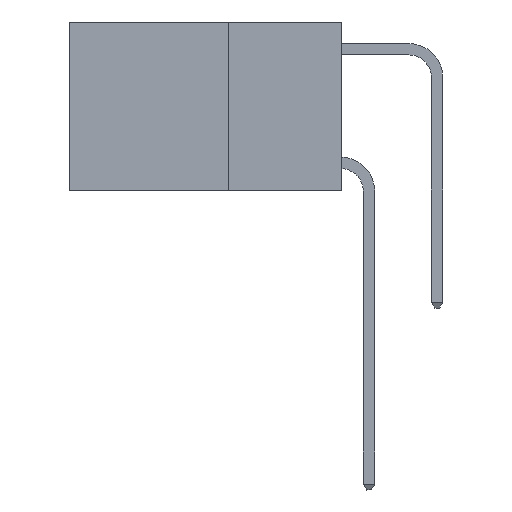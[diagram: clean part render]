
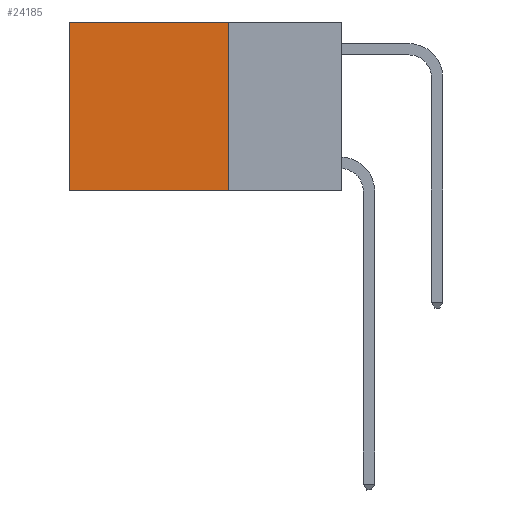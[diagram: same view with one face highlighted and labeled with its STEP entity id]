
A CAD part, left-side view. The second image highlights one B-rep face of the part: STEP entity #24185.
In plain terms, the highlighted planar face has unit normal (-1, 0, 0).
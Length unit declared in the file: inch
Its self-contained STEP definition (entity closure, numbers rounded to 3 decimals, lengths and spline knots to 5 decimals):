
#81 = CARTESIAN_POINT ( 'NONE',  ( 0.2625, 0.6, -0.37 ) ) ;
#1152 = ORIENTED_EDGE ( 'NONE', *, *, #24016, .T. ) ;
#2086 = VECTOR ( 'NONE', #6227, 39.37008 ) ;
#2384 = VERTEX_POINT ( 'NONE', #5807 ) ;
#2871 = CARTESIAN_POINT ( 'NONE',  ( 0.2625, 0.25, 0. ) ) ;
#3083 = EDGE_LOOP ( 'NONE', ( #29100, #20463, #23077, #1152 ) ) ;
#3670 = VECTOR ( 'NONE', #8226, 39.37008 ) ;
#3983 = LINE ( 'NONE', #14456, #13531 ) ;
#4513 = VERTEX_POINT ( 'NONE', #81 ) ;
#5807 = CARTESIAN_POINT ( 'NONE',  ( 0.2625, 0.25, 0. ) ) ;
#6227 = DIRECTION ( 'NONE',  ( 0., 1., 0. ) ) ;
#7816 = LINE ( 'NONE', #2871, #2086 ) ;
#7934 = LINE ( 'NONE', #18418, #25900 ) ;
#8226 = DIRECTION ( 'NONE',  ( 0., 1., 0. ) ) ;
#9347 = EDGE_CURVE ( 'NONE', #2384, #14839, #3983, .T. ) ;
#10185 = VERTEX_POINT ( 'NONE', #24954 ) ;
#10388 = CARTESIAN_POINT ( 'NONE',  ( 0.2625, 0.25, -0.37 ) ) ;
#10631 = CARTESIAN_POINT ( 'NONE',  ( 0.2625, 0.25, -0.37 ) ) ;
#11155 = LINE ( 'NONE', #10631, #3670 ) ;
#11857 = DIRECTION ( 'NONE',  ( 0., 0., -1. ) ) ;
#13272 = DIRECTION ( 'NONE',  ( 0., 0., -1. ) ) ;
#13531 = VECTOR ( 'NONE', #11857, 39.37008 ) ;
#14456 = CARTESIAN_POINT ( 'NONE',  ( 0.2625, 0.25, 0. ) ) ;
#14839 = VERTEX_POINT ( 'NONE', #10388 ) ;
#15429 = EDGE_CURVE ( 'NONE', #10185, #4513, #7934, .T. ) ;
#16340 = AXIS2_PLACEMENT_3D ( 'NONE', #16878, #24934, #19444 ) ;
#16878 = CARTESIAN_POINT ( 'NONE',  ( 0.2625, 0.25, 0. ) ) ;
#18418 = CARTESIAN_POINT ( 'NONE',  ( 0.2625, 0.6, 0. ) ) ;
#19444 = DIRECTION ( 'NONE',  ( 0., 0., -1. ) ) ;
#20463 = ORIENTED_EDGE ( 'NONE', *, *, #23009, .F. ) ;
#23009 = EDGE_CURVE ( 'NONE', #14839, #4513, #11155, .T. ) ;
#23077 = ORIENTED_EDGE ( 'NONE', *, *, #9347, .F. ) ;
#24016 = EDGE_CURVE ( 'NONE', #2384, #10185, #7816, .T. ) ;
#24185 = ADVANCED_FACE ( 'NONE', ( #27657 ), #32922, .F. ) ;
#24934 = DIRECTION ( 'NONE',  ( 1., 0., 0. ) ) ;
#24954 = CARTESIAN_POINT ( 'NONE',  ( 0.2625, 0.6, 0. ) ) ;
#25900 = VECTOR ( 'NONE', #13272, 39.37008 ) ;
#27657 = FACE_OUTER_BOUND ( 'NONE', #3083, .T. ) ;
#29100 = ORIENTED_EDGE ( 'NONE', *, *, #15429, .T. ) ;
#32922 = PLANE ( 'NONE',  #16340 ) ;
